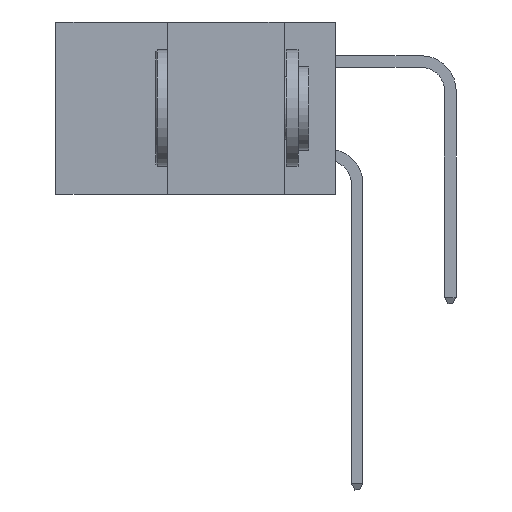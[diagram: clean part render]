
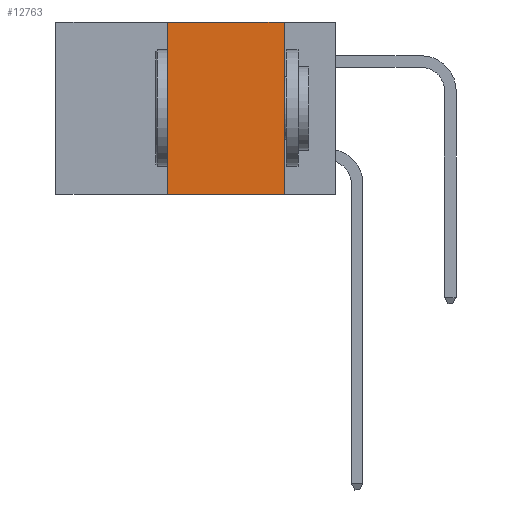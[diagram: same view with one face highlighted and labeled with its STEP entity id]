
A CAD part, left-side view. The second image highlights one B-rep face of the part: STEP entity #12763.
In plain terms, the highlighted planar face has unit normal (-1, 0, 0).
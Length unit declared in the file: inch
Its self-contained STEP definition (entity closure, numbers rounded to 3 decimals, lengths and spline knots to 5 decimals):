
#999 = LINE ( 'NONE', #15483, #13453 ) ;
#1415 = CARTESIAN_POINT ( 'NONE',  ( 0., 0.11, -0.37 ) ) ;
#1493 = EDGE_CURVE ( 'NONE', #16660, #13874, #8644, .T. ) ;
#1648 = DIRECTION ( 'NONE',  ( 0., -1., 0. ) ) ;
#1696 = VERTEX_POINT ( 'NONE', #13665 ) ;
#2604 = DIRECTION ( 'NONE',  ( 0., 0., 1. ) ) ;
#3126 = CARTESIAN_POINT ( 'NONE',  ( 0., 0.36, 0. ) ) ;
#3276 = EDGE_LOOP ( 'NONE', ( #13530, #13152, #13095, #13019 ) ) ;
#6379 = VECTOR ( 'NONE', #2604, 39.37008 ) ;
#6874 = LINE ( 'NONE', #13421, #6379 ) ;
#7148 = FACE_OUTER_BOUND ( 'NONE', #3276, .T. ) ;
#8059 = CARTESIAN_POINT ( 'NONE',  ( 0., 0.6, 0. ) ) ;
#8644 = LINE ( 'NONE', #11426, #19389 ) ;
#9582 = DIRECTION ( 'NONE',  ( 0., 0., -1. ) ) ;
#10243 = EDGE_CURVE ( 'NONE', #11560, #1696, #16674, .T. ) ;
#10619 = CARTESIAN_POINT ( 'NONE',  ( 0., 0.6, 0. ) ) ;
#11044 = DIRECTION ( 'NONE',  ( 0., 0., -1. ) ) ;
#11426 = CARTESIAN_POINT ( 'NONE',  ( 0., 0.6, -0.37 ) ) ;
#11560 = VERTEX_POINT ( 'NONE', #3126 ) ;
#11621 = EDGE_CURVE ( 'NONE', #1696, #13874, #999, .T. ) ;
#12009 = EDGE_CURVE ( 'NONE', #16660, #11560, #6874, .T. ) ;
#12367 = VECTOR ( 'NONE', #16454, 39.37008 ) ;
#12763 = ADVANCED_FACE ( 'NONE', ( #7148 ), #13989, .F. ) ;
#13019 = ORIENTED_EDGE ( 'NONE', *, *, #1493, .T. ) ;
#13095 = ORIENTED_EDGE ( 'NONE', *, *, #12009, .F. ) ;
#13152 = ORIENTED_EDGE ( 'NONE', *, *, #10243, .F. ) ;
#13421 = CARTESIAN_POINT ( 'NONE',  ( 0., 0.36, 0. ) ) ;
#13453 = VECTOR ( 'NONE', #11044, 39.37008 ) ;
#13530 = ORIENTED_EDGE ( 'NONE', *, *, #11621, .F. ) ;
#13665 = CARTESIAN_POINT ( 'NONE',  ( 0., 0.11, 0. ) ) ;
#13874 = VERTEX_POINT ( 'NONE', #1415 ) ;
#13989 = PLANE ( 'NONE',  #19466 ) ;
#14785 = CARTESIAN_POINT ( 'NONE',  ( 0., 0.36, -0.37 ) ) ;
#15483 = CARTESIAN_POINT ( 'NONE',  ( 0., 0.11, 0. ) ) ;
#16454 = DIRECTION ( 'NONE',  ( 0., -1., 0. ) ) ;
#16660 = VERTEX_POINT ( 'NONE', #14785 ) ;
#16674 = LINE ( 'NONE', #10619, #12367 ) ;
#18335 = DIRECTION ( 'NONE',  ( 1., 0., 0. ) ) ;
#19389 = VECTOR ( 'NONE', #1648, 39.37008 ) ;
#19466 = AXIS2_PLACEMENT_3D ( 'NONE', #8059, #18335, #9582 ) ;
